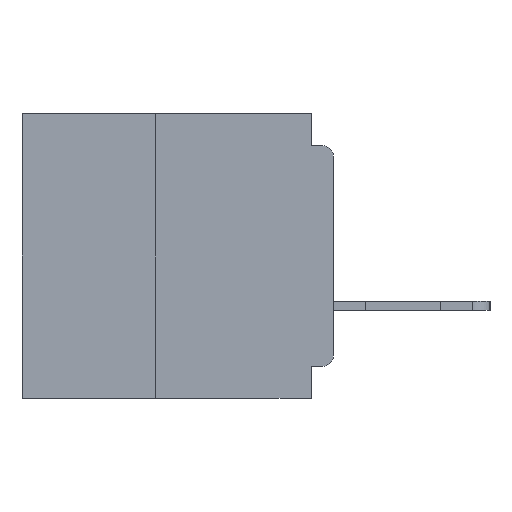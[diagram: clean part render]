
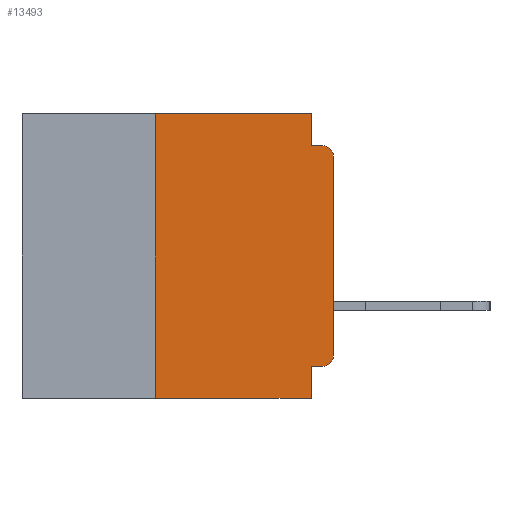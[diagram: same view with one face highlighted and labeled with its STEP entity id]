
A CAD part, left-side view. The second image highlights one B-rep face of the part: STEP entity #13493.
In plain terms, the highlighted planar face has unit normal (-1, 0, 0).
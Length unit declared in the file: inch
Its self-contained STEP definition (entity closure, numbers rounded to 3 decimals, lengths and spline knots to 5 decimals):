
#180 = DIRECTION ( 'NONE',  ( 0., 0., -1. ) ) ;
#360 = AXIS2_PLACEMENT_3D ( 'NONE', #462, #22450, #3614 ) ;
#462 = CARTESIAN_POINT ( 'NONE',  ( 0., 0.015, -0.34 ) ) ;
#1770 = VECTOR ( 'NONE', #18340, 39.37008 ) ;
#2805 = CARTESIAN_POINT ( 'NONE',  ( 0., 0.437, 0. ) ) ;
#3331 = VERTEX_POINT ( 'NONE', #12992 ) ;
#3423 = EDGE_CURVE ( 'NONE', #20818, #3331, #8210, .T. ) ;
#3614 = DIRECTION ( 'NONE',  ( 0., 0., -1. ) ) ;
#5499 = CARTESIAN_POINT ( 'NONE',  ( 0., 0.015, -0.355 ) ) ;
#5938 = LINE ( 'NONE', #34142, #38202 ) ;
#5962 = DIRECTION ( 'NONE',  ( 0., 0., -1. ) ) ;
#6049 = EDGE_CURVE ( 'NONE', #31268, #12096, #7035, .T. ) ;
#6373 = VERTEX_POINT ( 'NONE', #8194 ) ;
#6757 = CARTESIAN_POINT ( 'NONE',  ( 0., 0.015, -0.06 ) ) ;
#7035 = CIRCLE ( 'NONE', #39055, 0.015 ) ;
#7152 = CARTESIAN_POINT ( 'NONE',  ( 0., 0., -0.045 ) ) ;
#7168 = VECTOR ( 'NONE', #8350, 39.37008 ) ;
#7386 = VERTEX_POINT ( 'NONE', #38069 ) ;
#8194 = CARTESIAN_POINT ( 'NONE',  ( 0., 0.031, -0.4 ) ) ;
#8210 = LINE ( 'NONE', #9939, #25915 ) ;
#8350 = DIRECTION ( 'NONE',  ( 0., -1., 0. ) ) ;
#8534 = CARTESIAN_POINT ( 'NONE',  ( 0., 0.25, 0. ) ) ;
#8750 = VERTEX_POINT ( 'NONE', #5499 ) ;
#9362 = VERTEX_POINT ( 'NONE', #30502 ) ;
#9848 = DIRECTION ( 'NONE',  ( 0., 0., -1. ) ) ;
#9939 = CARTESIAN_POINT ( 'NONE',  ( 0., 0.031, 0. ) ) ;
#10215 = EDGE_CURVE ( 'NONE', #30874, #6373, #29756, .T. ) ;
#10371 = CARTESIAN_POINT ( 'NONE',  ( 0., 0.031, -0.355 ) ) ;
#10597 = DIRECTION ( 'NONE',  ( 0., 0., -1. ) ) ;
#10838 = ORIENTED_EDGE ( 'NONE', *, *, #15298, .F. ) ;
#11017 = ORIENTED_EDGE ( 'NONE', *, *, #6049, .T. ) ;
#11999 = ORIENTED_EDGE ( 'NONE', *, *, #3423, .F. ) ;
#12096 = VERTEX_POINT ( 'NONE', #19575 ) ;
#12112 = PLANE ( 'NONE',  #38459 ) ;
#12597 = DIRECTION ( 'NONE',  ( 0., -1., 0. ) ) ;
#12992 = CARTESIAN_POINT ( 'NONE',  ( 0., 0.031, -0.045 ) ) ;
#13311 = ORIENTED_EDGE ( 'NONE', *, *, #10215, .F. ) ;
#13409 = VERTEX_POINT ( 'NONE', #8534 ) ;
#13493 = ADVANCED_FACE ( 'NONE', ( #20314 ), #12112, .F. ) ;
#13976 = ORIENTED_EDGE ( 'NONE', *, *, #31992, .T. ) ;
#14016 = ORIENTED_EDGE ( 'NONE', *, *, #27056, .F. ) ;
#14484 = EDGE_CURVE ( 'NONE', #8750, #30874, #25565, .T. ) ;
#14694 = DIRECTION ( 'NONE',  ( 0., 1., 0. ) ) ;
#15174 = CARTESIAN_POINT ( 'NONE',  ( 0., 0., 0. ) ) ;
#15298 = EDGE_CURVE ( 'NONE', #7386, #13409, #5938, .T. ) ;
#15558 = LINE ( 'NONE', #30154, #7168 ) ;
#16275 = ORIENTED_EDGE ( 'NONE', *, *, #25759, .T. ) ;
#16509 = CIRCLE ( 'NONE', #360, 0.015 ) ;
#17260 = VECTOR ( 'NONE', #12597, 39.37008 ) ;
#17934 = EDGE_CURVE ( 'NONE', #9362, #31268, #26769, .T. ) ;
#18340 = DIRECTION ( 'NONE',  ( 0., 0., 1. ) ) ;
#18887 = EDGE_LOOP ( 'NONE', ( #27978, #11017, #14016, #11999, #30072, #10838, #16275, #13311, #39678, #13976 ) ) ;
#19575 = CARTESIAN_POINT ( 'NONE',  ( 0., 0.015, -0.045 ) ) ;
#20314 = FACE_OUTER_BOUND ( 'NONE', #18887, .T. ) ;
#20818 = VERTEX_POINT ( 'NONE', #21642 ) ;
#21642 = CARTESIAN_POINT ( 'NONE',  ( 0., 0.031, 0. ) ) ;
#21830 = CARTESIAN_POINT ( 'NONE',  ( 0., 0., -0.06 ) ) ;
#22450 = DIRECTION ( 'NONE',  ( -1., 0., 0. ) ) ;
#24251 = LINE ( 'NONE', #7152, #31530 ) ;
#24764 = DIRECTION ( 'NONE',  ( 1., 0., 0. ) ) ;
#25565 = LINE ( 'NONE', #33390, #33845 ) ;
#25567 = LINE ( 'NONE', #28214, #17260 ) ;
#25759 = EDGE_CURVE ( 'NONE', #7386, #6373, #25567, .T. ) ;
#25915 = VECTOR ( 'NONE', #10597, 39.37008 ) ;
#26769 = LINE ( 'NONE', #15174, #1770 ) ;
#27056 = EDGE_CURVE ( 'NONE', #3331, #12096, #24251, .T. ) ;
#27978 = ORIENTED_EDGE ( 'NONE', *, *, #17934, .T. ) ;
#28214 = CARTESIAN_POINT ( 'NONE',  ( 0., 0.437, -0.4 ) ) ;
#28662 = DIRECTION ( 'NONE',  ( -1., 0., 0. ) ) ;
#28797 = VECTOR ( 'NONE', #180, 39.37008 ) ;
#29756 = LINE ( 'NONE', #34510, #28797 ) ;
#30072 = ORIENTED_EDGE ( 'NONE', *, *, #40338, .F. ) ;
#30154 = CARTESIAN_POINT ( 'NONE',  ( 0., 0.437, 0. ) ) ;
#30502 = CARTESIAN_POINT ( 'NONE',  ( 0., 0., -0.34 ) ) ;
#30874 = VERTEX_POINT ( 'NONE', #10371 ) ;
#31268 = VERTEX_POINT ( 'NONE', #21830 ) ;
#31530 = VECTOR ( 'NONE', #32062, 39.37008 ) ;
#31992 = EDGE_CURVE ( 'NONE', #8750, #9362, #16509, .T. ) ;
#32062 = DIRECTION ( 'NONE',  ( 0., -1., 0. ) ) ;
#33390 = CARTESIAN_POINT ( 'NONE',  ( 0., 0., -0.355 ) ) ;
#33845 = VECTOR ( 'NONE', #14694, 39.37008 ) ;
#34142 = CARTESIAN_POINT ( 'NONE',  ( 0., 0.25, -0.4 ) ) ;
#34510 = CARTESIAN_POINT ( 'NONE',  ( 0., 0.031, -0.4 ) ) ;
#38069 = CARTESIAN_POINT ( 'NONE',  ( 0., 0.25, -0.4 ) ) ;
#38202 = VECTOR ( 'NONE', #40348, 39.37008 ) ;
#38459 = AXIS2_PLACEMENT_3D ( 'NONE', #2805, #24764, #5962 ) ;
#39055 = AXIS2_PLACEMENT_3D ( 'NONE', #6757, #28662, #9848 ) ;
#39678 = ORIENTED_EDGE ( 'NONE', *, *, #14484, .F. ) ;
#40338 = EDGE_CURVE ( 'NONE', #13409, #20818, #15558, .T. ) ;
#40348 = DIRECTION ( 'NONE',  ( 0., 0., 1. ) ) ;
